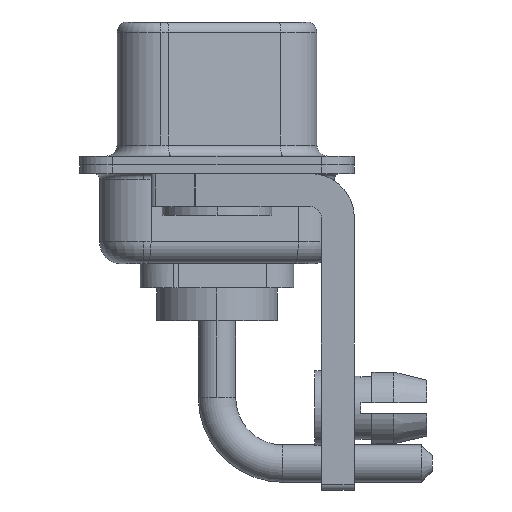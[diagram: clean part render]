
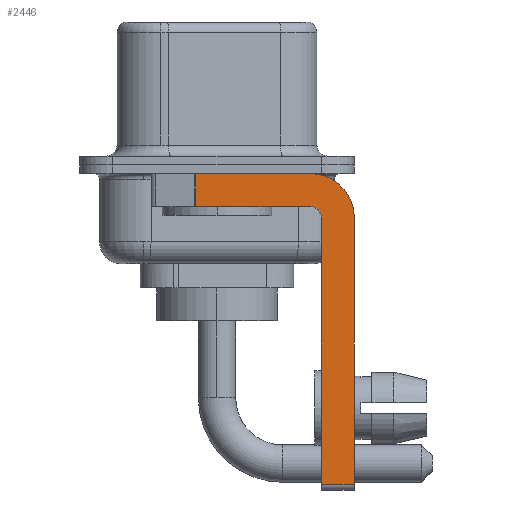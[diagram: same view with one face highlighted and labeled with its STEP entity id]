
A CAD part, left-side view. The second image highlights one B-rep face of the part: STEP entity #2446.
In plain terms, the highlighted planar face has unit normal (-1, 0, 0).
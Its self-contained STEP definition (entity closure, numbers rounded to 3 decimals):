
#74 = CARTESIAN_POINT ( 'NONE',  ( -2.9, -4.25, -2.4 ) ) ;
#144 = CARTESIAN_POINT ( 'NONE',  ( -2.9, 0.978, -1.9 ) ) ;
#156 = VERTEX_POINT ( 'NONE', #144 ) ;
#430 = ORIENTED_EDGE ( 'NONE', *, *, #12966, .F. ) ;
#491 = VERTEX_POINT ( 'NONE', #16563 ) ;
#1153 = LINE ( 'NONE', #10783, #14443 ) ;
#1520 = VERTEX_POINT ( 'NONE', #14637 ) ;
#2187 = ORIENTED_EDGE ( 'NONE', *, *, #11035, .F. ) ;
#2362 = DIRECTION ( 'NONE',  ( -1., 0., 0. ) ) ;
#2446 = ADVANCED_FACE ( 'NONE', ( #7197 ), #5837, .F. ) ;
#2569 = EDGE_CURVE ( 'NONE', #11416, #1520, #10445, .T. ) ;
#2618 = VECTOR ( 'NONE', #15765, 1000. ) ;
#2874 = ORIENTED_EDGE ( 'NONE', *, *, #11729, .F. ) ;
#3112 = AXIS2_PLACEMENT_3D ( 'NONE', #17531, #2362, #10391 ) ;
#3191 = ORIENTED_EDGE ( 'NONE', *, *, #2569, .F. ) ;
#4694 = LINE ( 'NONE', #10230, #5438 ) ;
#5438 = VECTOR ( 'NONE', #12708, 1000. ) ;
#5837 = PLANE ( 'NONE',  #15808 ) ;
#6185 = VECTOR ( 'NONE', #6687, 1000. ) ;
#6687 = DIRECTION ( 'NONE',  ( 0., 1., 0. ) ) ;
#6875 = VECTOR ( 'NONE', #9242, 1000. ) ;
#6877 = CARTESIAN_POINT ( 'NONE',  ( -2.9, -4.25, -1.9 ) ) ;
#7197 = FACE_OUTER_BOUND ( 'NONE', #7786, .T. ) ;
#7702 = AXIS2_PLACEMENT_3D ( 'NONE', #17854, #14644, #10615 ) ;
#7703 = ORIENTED_EDGE ( 'NONE', *, *, #11702, .T. ) ;
#7786 = EDGE_LOOP ( 'NONE', ( #2187, #14797, #13065, #430, #3191, #7703, #2874, #15182 ) ) ;
#8000 = VECTOR ( 'NONE', #15598, 1000. ) ;
#8963 = CARTESIAN_POINT ( 'NONE',  ( -2.9, -4.25, -0.4 ) ) ;
#9242 = DIRECTION ( 'NONE',  ( 0., -1., 0. ) ) ;
#9744 = CIRCLE ( 'NONE', #7702, 2. ) ;
#9745 = DIRECTION ( 'NONE',  ( 1., 0., 0. ) ) ;
#10017 = CARTESIAN_POINT ( 'NONE',  ( -2.9, 3., -0.4 ) ) ;
#10181 = VERTEX_POINT ( 'NONE', #8963 ) ;
#10230 = CARTESIAN_POINT ( 'NONE',  ( -2.9, 0.978, -1.9 ) ) ;
#10391 = DIRECTION ( 'NONE',  ( 0., 0., 1. ) ) ;
#10445 = LINE ( 'NONE', #16023, #2618 ) ;
#10615 = DIRECTION ( 'NONE',  ( 0., 0., -1. ) ) ;
#10687 = LINE ( 'NONE', #6877, #6185 ) ;
#10696 = CARTESIAN_POINT ( 'NONE',  ( -2.9, -4.25, -14.55 ) ) ;
#10783 = CARTESIAN_POINT ( 'NONE',  ( -2.9, -6.25, -2.4 ) ) ;
#10967 = CIRCLE ( 'NONE', #3112, 0.5 ) ;
#11035 = EDGE_CURVE ( 'NONE', #11895, #10181, #18083, .T. ) ;
#11184 = CARTESIAN_POINT ( 'NONE',  ( -2.9, -4.75, -14.55 ) ) ;
#11416 = VERTEX_POINT ( 'NONE', #11184 ) ;
#11478 = DIRECTION ( 'NONE',  ( 0., 0., -1. ) ) ;
#11702 = EDGE_CURVE ( 'NONE', #11416, #17789, #16001, .T. ) ;
#11729 = EDGE_CURVE ( 'NONE', #491, #17789, #1153, .T. ) ;
#11895 = VERTEX_POINT ( 'NONE', #18040 ) ;
#12044 = EDGE_CURVE ( 'NONE', #11895, #156, #4694, .T. ) ;
#12708 = DIRECTION ( 'NONE',  ( 0., 0., -1. ) ) ;
#12966 = EDGE_CURVE ( 'NONE', #1520, #13903, #10967, .T. ) ;
#13065 = ORIENTED_EDGE ( 'NONE', *, *, #15363, .F. ) ;
#13758 = CARTESIAN_POINT ( 'NONE',  ( -2.9, -4.25, -1.9 ) ) ;
#13903 = VERTEX_POINT ( 'NONE', #13758 ) ;
#14443 = VECTOR ( 'NONE', #17572, 1000. ) ;
#14637 = CARTESIAN_POINT ( 'NONE',  ( -2.9, -4.75, -2.4 ) ) ;
#14644 = DIRECTION ( 'NONE',  ( 1., 0., 0. ) ) ;
#14797 = ORIENTED_EDGE ( 'NONE', *, *, #12044, .T. ) ;
#15182 = ORIENTED_EDGE ( 'NONE', *, *, #17996, .F. ) ;
#15363 = EDGE_CURVE ( 'NONE', #13903, #156, #10687, .T. ) ;
#15598 = DIRECTION ( 'NONE',  ( 0., -1., 0. ) ) ;
#15749 = CARTESIAN_POINT ( 'NONE',  ( -2.9, -6.25, -14.55 ) ) ;
#15765 = DIRECTION ( 'NONE',  ( 0., 0., 1. ) ) ;
#15808 = AXIS2_PLACEMENT_3D ( 'NONE', #74, #9745, #11478 ) ;
#16001 = LINE ( 'NONE', #10696, #6875 ) ;
#16023 = CARTESIAN_POINT ( 'NONE',  ( -2.9, -4.75, -14.8 ) ) ;
#16563 = CARTESIAN_POINT ( 'NONE',  ( -2.9, -6.25, -2.4 ) ) ;
#17531 = CARTESIAN_POINT ( 'NONE',  ( -2.9, -4.25, -2.4 ) ) ;
#17572 = DIRECTION ( 'NONE',  ( 0., 0., -1. ) ) ;
#17789 = VERTEX_POINT ( 'NONE', #15749 ) ;
#17854 = CARTESIAN_POINT ( 'NONE',  ( -2.9, -4.25, -2.4 ) ) ;
#17996 = EDGE_CURVE ( 'NONE', #10181, #491, #9744, .T. ) ;
#18040 = CARTESIAN_POINT ( 'NONE',  ( -2.9, 0.978, -0.4 ) ) ;
#18083 = LINE ( 'NONE', #10017, #8000 ) ;
